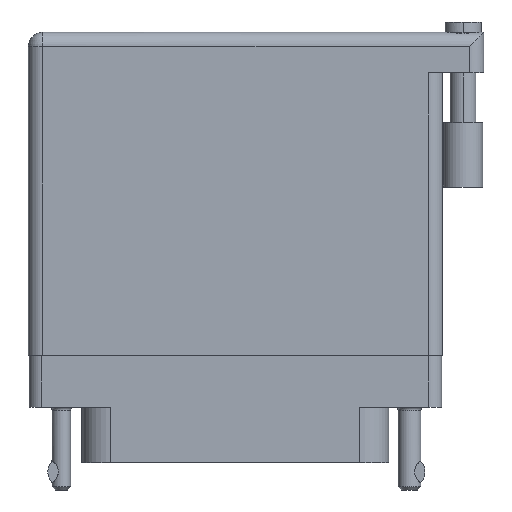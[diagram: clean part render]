
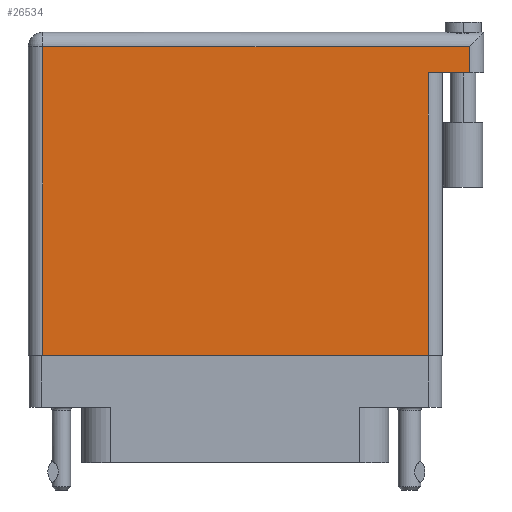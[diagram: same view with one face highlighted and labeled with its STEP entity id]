
A CAD part, front view. The second image highlights one B-rep face of the part: STEP entity #26534.
In plain terms, the highlighted face is planar.
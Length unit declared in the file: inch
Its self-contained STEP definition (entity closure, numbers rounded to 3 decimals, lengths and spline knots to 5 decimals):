
#470 = DIRECTION ( 'NONE',  ( 0., 1., 0. ) ) ;
#1217 = CARTESIAN_POINT ( 'NONE',  ( 0.934, -0.1, 0.4495 ) ) ;
#2634 = EDGE_CURVE ( 'NONE', #38391, #32545, #4123, .T. ) ;
#3376 = DIRECTION ( 'NONE',  ( 0., 0., -1. ) ) ;
#3439 = VERTEX_POINT ( 'NONE', #18469 ) ;
#3528 = CARTESIAN_POINT ( 'NONE',  ( -1.004, 1.466, 0.4495 ) ) ;
#3703 = VERTEX_POINT ( 'NONE', #16433 ) ;
#3836 = DIRECTION ( 'NONE',  ( 0., 1., 0. ) ) ;
#4028 = EDGE_CURVE ( 'NONE', #41896, #38391, #32845, .T. ) ;
#4123 = LINE ( 'NONE', #38935, #16599 ) ;
#5637 = DIRECTION ( 'NONE',  ( -1., 0., 0. ) ) ;
#6170 = LINE ( 'NONE', #20009, #27327 ) ;
#6433 = PLANE ( 'NONE',  #32077 ) ;
#6529 = EDGE_CURVE ( 'NONE', #20630, #3703, #6170, .T. ) ;
#6629 = FACE_OUTER_BOUND ( 'NONE', #15684, .T. ) ;
#9058 = DIRECTION ( 'NONE',  ( 0., -1., 0. ) ) ;
#9096 = CARTESIAN_POINT ( 'NONE',  ( -1.004, 1.396, 0.4495 ) ) ;
#9685 = CARTESIAN_POINT ( 'NONE',  ( -0.934, -0.1, 0.4495 ) ) ;
#10094 = EDGE_CURVE ( 'NONE', #3439, #41896, #12877, .T. ) ;
#12877 = LINE ( 'NONE', #9096, #29235 ) ;
#14095 = CARTESIAN_POINT ( 'NONE',  ( 1.134, 1.269, 0.4495 ) ) ;
#15684 = EDGE_LOOP ( 'NONE', ( #23302, #20194, #43407, #16522, #38676, #24869 ) ) ;
#16433 = CARTESIAN_POINT ( 'NONE',  ( 0.934, 1.269, 0.4495 ) ) ;
#16522 = ORIENTED_EDGE ( 'NONE', *, *, #34676, .T. ) ;
#16599 = VECTOR ( 'NONE', #35862, 39.37008 ) ;
#16914 = CARTESIAN_POINT ( 'NONE',  ( 0.934, 1.269, 0.4495 ) ) ;
#18469 = CARTESIAN_POINT ( 'NONE',  ( 1.134, 1.396, 0.4495 ) ) ;
#20009 = CARTESIAN_POINT ( 'NONE',  ( 1.204, 1.269, 0.4495 ) ) ;
#20194 = ORIENTED_EDGE ( 'NONE', *, *, #43225, .T. ) ;
#20325 = VECTOR ( 'NONE', #9058, 39.37008 ) ;
#20556 = VECTOR ( 'NONE', #3836, 39.37008 ) ;
#20630 = VERTEX_POINT ( 'NONE', #14095 ) ;
#20694 = CARTESIAN_POINT ( 'NONE',  ( 1.134, 1.466, 0.4495 ) ) ;
#20881 = DIRECTION ( 'NONE',  ( -1., 0., 0. ) ) ;
#23195 = CARTESIAN_POINT ( 'NONE',  ( -0.934, -0.1, 0.4495 ) ) ;
#23302 = ORIENTED_EDGE ( 'NONE', *, *, #2634, .T. ) ;
#24869 = ORIENTED_EDGE ( 'NONE', *, *, #4028, .T. ) ;
#26534 = ADVANCED_FACE ( 'NONE', ( #6629 ), #6433, .F. ) ;
#27327 = VECTOR ( 'NONE', #20881, 39.37008 ) ;
#29235 = VECTOR ( 'NONE', #5637, 39.37008 ) ;
#32077 = AXIS2_PLACEMENT_3D ( 'NONE', #3528, #3376, #34507 ) ;
#32469 = LINE ( 'NONE', #20694, #38447 ) ;
#32545 = VERTEX_POINT ( 'NONE', #1217 ) ;
#32845 = LINE ( 'NONE', #23195, #20325 ) ;
#34507 = DIRECTION ( 'NONE',  ( -1., 0., 0. ) ) ;
#34676 = EDGE_CURVE ( 'NONE', #20630, #3439, #32469, .T. ) ;
#35862 = DIRECTION ( 'NONE',  ( 1., 0., 0. ) ) ;
#36182 = CARTESIAN_POINT ( 'NONE',  ( -0.934, 1.396, 0.4495 ) ) ;
#38391 = VERTEX_POINT ( 'NONE', #9685 ) ;
#38447 = VECTOR ( 'NONE', #470, 39.37008 ) ;
#38480 = LINE ( 'NONE', #16914, #20556 ) ;
#38676 = ORIENTED_EDGE ( 'NONE', *, *, #10094, .T. ) ;
#38935 = CARTESIAN_POINT ( 'NONE',  ( -1.004, -0.1, 0.4495 ) ) ;
#41896 = VERTEX_POINT ( 'NONE', #36182 ) ;
#43225 = EDGE_CURVE ( 'NONE', #32545, #3703, #38480, .T. ) ;
#43407 = ORIENTED_EDGE ( 'NONE', *, *, #6529, .F. ) ;
